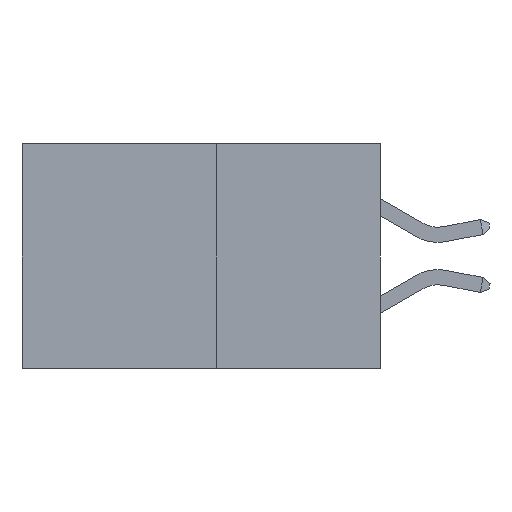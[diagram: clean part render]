
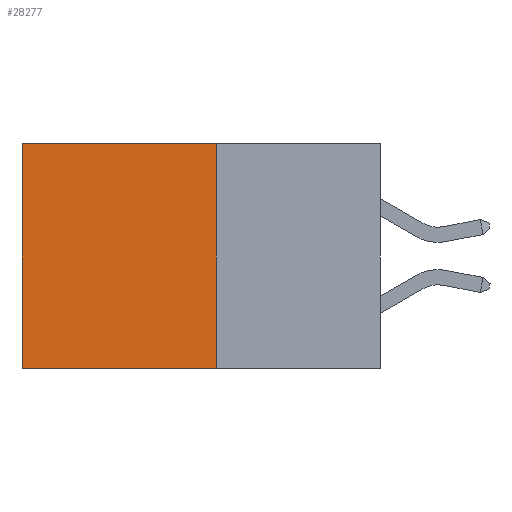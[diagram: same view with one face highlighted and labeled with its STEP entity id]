
A CAD part, left-side view. The second image highlights one B-rep face of the part: STEP entity #28277.
In plain terms, the highlighted planar face has unit normal (-1, 0, 0).
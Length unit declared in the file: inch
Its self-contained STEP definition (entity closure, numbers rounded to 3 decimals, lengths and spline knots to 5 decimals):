
#340 = AXIS2_PLACEMENT_3D ( 'NONE', #17054, #692, #19836 ) ;
#692 = DIRECTION ( 'NONE',  ( 1., 0., 0. ) ) ;
#1323 = ORIENTED_EDGE ( 'NONE', *, *, #34780, .F. ) ;
#5803 = VERTEX_POINT ( 'NONE', #31281 ) ;
#5829 = CARTESIAN_POINT ( 'NONE',  ( 0.277, 0.27, -0.37 ) ) ;
#7511 = VECTOR ( 'NONE', #8551, 39.37008 ) ;
#8123 = VECTOR ( 'NONE', #34535, 39.37008 ) ;
#8510 = LINE ( 'NONE', #34460, #23056 ) ;
#8551 = DIRECTION ( 'NONE',  ( 0., 1., 0. ) ) ;
#9653 = LINE ( 'NONE', #16572, #16902 ) ;
#12751 = CARTESIAN_POINT ( 'NONE',  ( 0.277, 0.59, -0.37 ) ) ;
#13298 = CARTESIAN_POINT ( 'NONE',  ( 0.277, 0.59, -0.37 ) ) ;
#13896 = EDGE_CURVE ( 'NONE', #29151, #16543, #29340, .T. ) ;
#16543 = VERTEX_POINT ( 'NONE', #13298 ) ;
#16572 = CARTESIAN_POINT ( 'NONE',  ( 0.277, 0.27, -0.37 ) ) ;
#16902 = VECTOR ( 'NONE', #32980, 39.37008 ) ;
#17054 = CARTESIAN_POINT ( 'NONE',  ( 0.277, 0.27, -0.37 ) ) ;
#19836 = DIRECTION ( 'NONE',  ( 0., 0., -1. ) ) ;
#20614 = CARTESIAN_POINT ( 'NONE',  ( 0.277, 0.27, -0.37 ) ) ;
#23056 = VECTOR ( 'NONE', #26290, 39.37008 ) ;
#24382 = FACE_OUTER_BOUND ( 'NONE', #30662, .T. ) ;
#24548 = CARTESIAN_POINT ( 'NONE',  ( 0.277, 0.59, 0. ) ) ;
#25154 = ORIENTED_EDGE ( 'NONE', *, *, #29188, .T. ) ;
#26290 = DIRECTION ( 'NONE',  ( 0., 1., 0. ) ) ;
#27813 = EDGE_CURVE ( 'NONE', #28069, #16543, #29964, .T. ) ;
#28069 = VERTEX_POINT ( 'NONE', #24548 ) ;
#28277 = ADVANCED_FACE ( 'NONE', ( #24382 ), #33446, .F. ) ;
#29151 = VERTEX_POINT ( 'NONE', #20614 ) ;
#29188 = EDGE_CURVE ( 'NONE', #5803, #28069, #8510, .T. ) ;
#29340 = LINE ( 'NONE', #5829, #7511 ) ;
#29964 = LINE ( 'NONE', #12751, #8123 ) ;
#30662 = EDGE_LOOP ( 'NONE', ( #35336, #30979, #1323, #25154 ) ) ;
#30979 = ORIENTED_EDGE ( 'NONE', *, *, #13896, .F. ) ;
#31281 = CARTESIAN_POINT ( 'NONE',  ( 0.277, 0.27, 0. ) ) ;
#32980 = DIRECTION ( 'NONE',  ( 0., 0., -1. ) ) ;
#33446 = PLANE ( 'NONE',  #340 ) ;
#34460 = CARTESIAN_POINT ( 'NONE',  ( 0.277, 0.27, 0. ) ) ;
#34535 = DIRECTION ( 'NONE',  ( 0., 0., -1. ) ) ;
#34780 = EDGE_CURVE ( 'NONE', #5803, #29151, #9653, .T. ) ;
#35336 = ORIENTED_EDGE ( 'NONE', *, *, #27813, .T. ) ;
